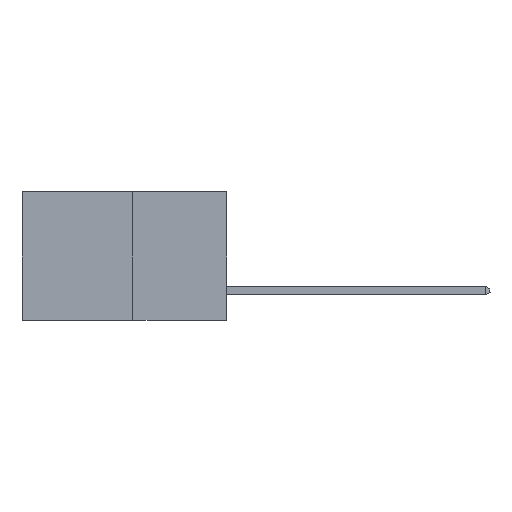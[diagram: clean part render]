
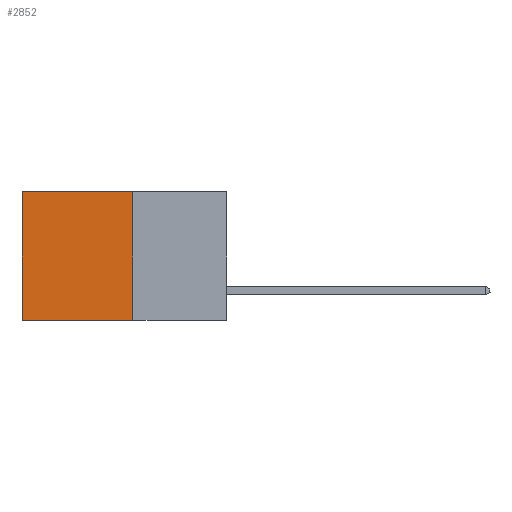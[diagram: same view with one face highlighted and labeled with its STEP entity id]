
A CAD part, left-side view. The second image highlights one B-rep face of the part: STEP entity #2852.
In plain terms, the highlighted planar face has unit normal (-1, 0, 0).
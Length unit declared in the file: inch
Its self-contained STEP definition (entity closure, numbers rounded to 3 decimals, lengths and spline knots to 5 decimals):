
#645 = CARTESIAN_POINT ( 'NONE',  ( 0.277, 0.59, -0.37 ) ) ;
#870 = DIRECTION ( 'NONE',  ( 0., 0., -1. ) ) ;
#997 = DIRECTION ( 'NONE',  ( 1., 0., 0. ) ) ;
#1045 = LINE ( 'NONE', #11611, #19572 ) ;
#1068 = CARTESIAN_POINT ( 'NONE',  ( 0.277, 0.27, -0.37 ) ) ;
#1072 = PLANE ( 'NONE',  #17442 ) ;
#1751 = EDGE_CURVE ( 'NONE', #11373, #15028, #1045, .T. ) ;
#1849 = CARTESIAN_POINT ( 'NONE',  ( 0.277, 0.27, 0. ) ) ;
#1898 = EDGE_LOOP ( 'NONE', ( #7248, #15237, #11906, #20212 ) ) ;
#2852 = ADVANCED_FACE ( 'NONE', ( #11650 ), #1072, .F. ) ;
#4002 = CARTESIAN_POINT ( 'NONE',  ( 0.277, 0.27, -0.37 ) ) ;
#5851 = CARTESIAN_POINT ( 'NONE',  ( 0.277, 0.27, -0.37 ) ) ;
#6550 = DIRECTION ( 'NONE',  ( 0., 1., 0. ) ) ;
#7248 = ORIENTED_EDGE ( 'NONE', *, *, #21855, .T. ) ;
#10062 = VERTEX_POINT ( 'NONE', #17801 ) ;
#11373 = VERTEX_POINT ( 'NONE', #1849 ) ;
#11383 = DIRECTION ( 'NONE',  ( 0., 0., -1. ) ) ;
#11611 = CARTESIAN_POINT ( 'NONE',  ( 0.277, 0.27, -0.37 ) ) ;
#11650 = FACE_OUTER_BOUND ( 'NONE', #1898, .T. ) ;
#11663 = DIRECTION ( 'NONE',  ( 0., 0., -1. ) ) ;
#11906 = ORIENTED_EDGE ( 'NONE', *, *, #1751, .F. ) ;
#14950 = LINE ( 'NONE', #20325, #18881 ) ;
#15028 = VERTEX_POINT ( 'NONE', #4002 ) ;
#15217 = VECTOR ( 'NONE', #11383, 39.37008 ) ;
#15237 = ORIENTED_EDGE ( 'NONE', *, *, #21791, .F. ) ;
#15740 = LINE ( 'NONE', #5851, #20195 ) ;
#15916 = CARTESIAN_POINT ( 'NONE',  ( 0.277, 0.59, -0.37 ) ) ;
#17442 = AXIS2_PLACEMENT_3D ( 'NONE', #1068, #997, #870 ) ;
#17801 = CARTESIAN_POINT ( 'NONE',  ( 0.277, 0.59, 0. ) ) ;
#18010 = DIRECTION ( 'NONE',  ( 0., 1., 0. ) ) ;
#18881 = VECTOR ( 'NONE', #6550, 39.37008 ) ;
#19572 = VECTOR ( 'NONE', #11663, 39.37008 ) ;
#19676 = LINE ( 'NONE', #645, #15217 ) ;
#20195 = VECTOR ( 'NONE', #18010, 39.37008 ) ;
#20212 = ORIENTED_EDGE ( 'NONE', *, *, #22070, .T. ) ;
#20325 = CARTESIAN_POINT ( 'NONE',  ( 0.277, 0.27, 0. ) ) ;
#21075 = VERTEX_POINT ( 'NONE', #15916 ) ;
#21791 = EDGE_CURVE ( 'NONE', #15028, #21075, #15740, .T. ) ;
#21855 = EDGE_CURVE ( 'NONE', #10062, #21075, #19676, .T. ) ;
#22070 = EDGE_CURVE ( 'NONE', #11373, #10062, #14950, .T. ) ;
